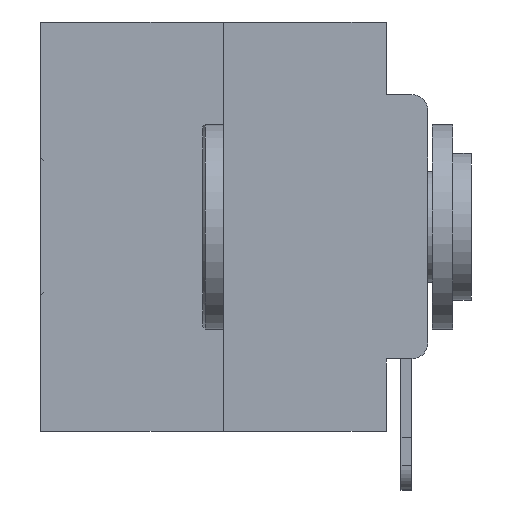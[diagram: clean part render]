
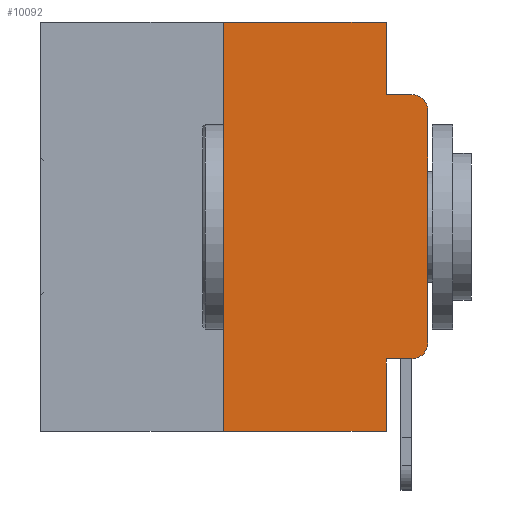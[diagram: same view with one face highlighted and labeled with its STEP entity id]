
A CAD part, left-side view. The second image highlights one B-rep face of the part: STEP entity #10092.
In plain terms, the highlighted planar face has unit normal (-1, 0, 0).
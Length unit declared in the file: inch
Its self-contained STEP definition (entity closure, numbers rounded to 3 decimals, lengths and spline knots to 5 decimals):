
#350 = DIRECTION ( 'NONE',  ( 0., 0., 1. ) ) ;
#868 = EDGE_CURVE ( 'NONE', #11809, #3276, #22494, .T. ) ;
#1090 = ORIENTED_EDGE ( 'NONE', *, *, #24768, .F. ) ;
#1964 = CARTESIAN_POINT ( 'NONE',  ( 0., 0.02, -0.3915 ) ) ;
#2411 = CARTESIAN_POINT ( 'NONE',  ( 0., 0.473, -0.5 ) ) ;
#2416 = ORIENTED_EDGE ( 'NONE', *, *, #868, .F. ) ;
#3276 = VERTEX_POINT ( 'NONE', #6260 ) ;
#3579 = CARTESIAN_POINT ( 'NONE',  ( 0., 0.051, -0.4115 ) ) ;
#4130 = LINE ( 'NONE', #23914, #23079 ) ;
#4134 = VERTEX_POINT ( 'NONE', #6064 ) ;
#4186 = DIRECTION ( 'NONE',  ( 0., 0., 1. ) ) ;
#4683 = VECTOR ( 'NONE', #15118, 39.37008 ) ;
#4741 = DIRECTION ( 'NONE',  ( 0., 0., -1. ) ) ;
#4911 = CIRCLE ( 'NONE', #29631, 0.02 ) ;
#5179 = DIRECTION ( 'NONE',  ( 1., 0., 0. ) ) ;
#5388 = CIRCLE ( 'NONE', #15864, 0.02 ) ;
#5958 = CARTESIAN_POINT ( 'NONE',  ( 0., 0.051, 0. ) ) ;
#6064 = CARTESIAN_POINT ( 'NONE',  ( 0., 0.051, -0.0885 ) ) ;
#6260 = CARTESIAN_POINT ( 'NONE',  ( 0., 0.051, -0.5 ) ) ;
#6265 = CARTESIAN_POINT ( 'NONE',  ( 0., 0.051, 0. ) ) ;
#6618 = ORIENTED_EDGE ( 'NONE', *, *, #16950, .T. ) ;
#6648 = ORIENTED_EDGE ( 'NONE', *, *, #8945, .F. ) ;
#6984 = EDGE_CURVE ( 'NONE', #27176, #3276, #11547, .T. ) ;
#7328 = DIRECTION ( 'NONE',  ( 0., -1., 0. ) ) ;
#8380 = EDGE_CURVE ( 'NONE', #11333, #25883, #5388, .T. ) ;
#8750 = EDGE_CURVE ( 'NONE', #11809, #11333, #16243, .T. ) ;
#8764 = ORIENTED_EDGE ( 'NONE', *, *, #24740, .F. ) ;
#8945 = EDGE_CURVE ( 'NONE', #31184, #14234, #16530, .T. ) ;
#9177 = VECTOR ( 'NONE', #15223, 39.37008 ) ;
#9835 = CARTESIAN_POINT ( 'NONE',  ( 0., 0.02, -0.4115 ) ) ;
#10092 = ADVANCED_FACE ( 'NONE', ( #20676 ), #27063, .F. ) ;
#10716 = ORIENTED_EDGE ( 'NONE', *, *, #8380, .T. ) ;
#11131 = VERTEX_POINT ( 'NONE', #23492 ) ;
#11333 = VERTEX_POINT ( 'NONE', #9835 ) ;
#11547 = LINE ( 'NONE', #2411, #4683 ) ;
#11809 = VERTEX_POINT ( 'NONE', #18744 ) ;
#12309 = AXIS2_PLACEMENT_3D ( 'NONE', #15125, #5179, #22404 ) ;
#13328 = ORIENTED_EDGE ( 'NONE', *, *, #8750, .T. ) ;
#13467 = DIRECTION ( 'NONE',  ( -1., 0., 0. ) ) ;
#14234 = VERTEX_POINT ( 'NONE', #5958 ) ;
#15118 = DIRECTION ( 'NONE',  ( 0., -1., 0. ) ) ;
#15125 = CARTESIAN_POINT ( 'NONE',  ( 0., 0.473, 0. ) ) ;
#15223 = DIRECTION ( 'NONE',  ( 0., 0., -1. ) ) ;
#15271 = VECTOR ( 'NONE', #350, 39.37008 ) ;
#15297 = DIRECTION ( 'NONE',  ( 0., -1., 0. ) ) ;
#15864 = AXIS2_PLACEMENT_3D ( 'NONE', #1964, #19576, #4741 ) ;
#16220 = DIRECTION ( 'NONE',  ( 0., -1., 0. ) ) ;
#16243 = LINE ( 'NONE', #3579, #27480 ) ;
#16530 = LINE ( 'NONE', #29051, #28502 ) ;
#16783 = LINE ( 'NONE', #22923, #15271 ) ;
#16950 = EDGE_CURVE ( 'NONE', #11131, #23719, #4911, .T. ) ;
#17550 = EDGE_CURVE ( 'NONE', #4134, #23719, #22989, .T. ) ;
#18536 = DIRECTION ( 'NONE',  ( 0., 0., -1. ) ) ;
#18572 = ORIENTED_EDGE ( 'NONE', *, *, #6984, .T. ) ;
#18744 = CARTESIAN_POINT ( 'NONE',  ( 0., 0.051, -0.4115 ) ) ;
#19576 = DIRECTION ( 'NONE',  ( -1., 0., 0. ) ) ;
#19579 = EDGE_CURVE ( 'NONE', #25883, #11131, #4130, .T. ) ;
#20676 = FACE_OUTER_BOUND ( 'NONE', #26181, .T. ) ;
#21173 = ORIENTED_EDGE ( 'NONE', *, *, #17550, .F. ) ;
#21515 = CARTESIAN_POINT ( 'NONE',  ( 0., 0.02, -0.0885 ) ) ;
#21932 = CARTESIAN_POINT ( 'NONE',  ( 0., 0.25, 0. ) ) ;
#22404 = DIRECTION ( 'NONE',  ( 0., 0., -1. ) ) ;
#22478 = CARTESIAN_POINT ( 'NONE',  ( 0., 0.051, -0.0885 ) ) ;
#22494 = LINE ( 'NONE', #6265, #28044 ) ;
#22923 = CARTESIAN_POINT ( 'NONE',  ( 0., 0.25, 0. ) ) ;
#22989 = LINE ( 'NONE', #22478, #28546 ) ;
#23079 = VECTOR ( 'NONE', #4186, 39.37008 ) ;
#23492 = CARTESIAN_POINT ( 'NONE',  ( 0., 0., -0.1085 ) ) ;
#23719 = VERTEX_POINT ( 'NONE', #21515 ) ;
#23787 = ORIENTED_EDGE ( 'NONE', *, *, #19579, .T. ) ;
#23914 = CARTESIAN_POINT ( 'NONE',  ( 0., 0., 0. ) ) ;
#24740 = EDGE_CURVE ( 'NONE', #14234, #4134, #28265, .T. ) ;
#24768 = EDGE_CURVE ( 'NONE', #27176, #31184, #16783, .T. ) ;
#25015 = CARTESIAN_POINT ( 'NONE',  ( 0., 0.25, -0.5 ) ) ;
#25883 = VERTEX_POINT ( 'NONE', #31931 ) ;
#26181 = EDGE_LOOP ( 'NONE', ( #23787, #6618, #21173, #8764, #6648, #1090, #18572, #2416, #13328, #10716 ) ) ;
#27063 = PLANE ( 'NONE',  #12309 ) ;
#27168 = CARTESIAN_POINT ( 'NONE',  ( 0., 0.051, 0. ) ) ;
#27176 = VERTEX_POINT ( 'NONE', #25015 ) ;
#27480 = VECTOR ( 'NONE', #16220, 39.37008 ) ;
#27793 = CARTESIAN_POINT ( 'NONE',  ( 0., 0.02, -0.1085 ) ) ;
#28044 = VECTOR ( 'NONE', #18536, 39.37008 ) ;
#28265 = LINE ( 'NONE', #27168, #9177 ) ;
#28502 = VECTOR ( 'NONE', #7328, 39.37008 ) ;
#28546 = VECTOR ( 'NONE', #15297, 39.37008 ) ;
#29051 = CARTESIAN_POINT ( 'NONE',  ( 0., 0.473, 0. ) ) ;
#29631 = AXIS2_PLACEMENT_3D ( 'NONE', #27793, #13467, #30134 ) ;
#30134 = DIRECTION ( 'NONE',  ( 0., 0., -1. ) ) ;
#31184 = VERTEX_POINT ( 'NONE', #21932 ) ;
#31931 = CARTESIAN_POINT ( 'NONE',  ( 0., 0., -0.3915 ) ) ;
